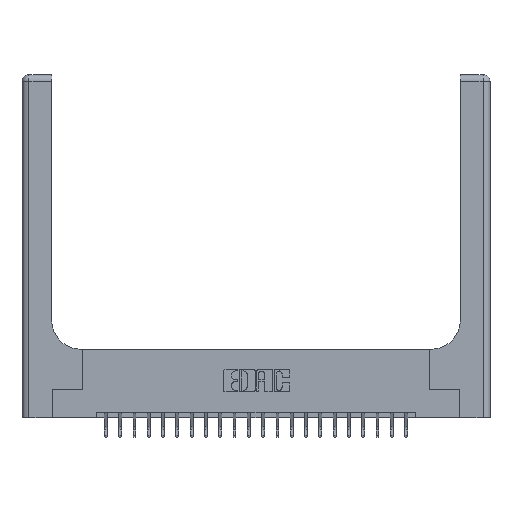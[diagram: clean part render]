
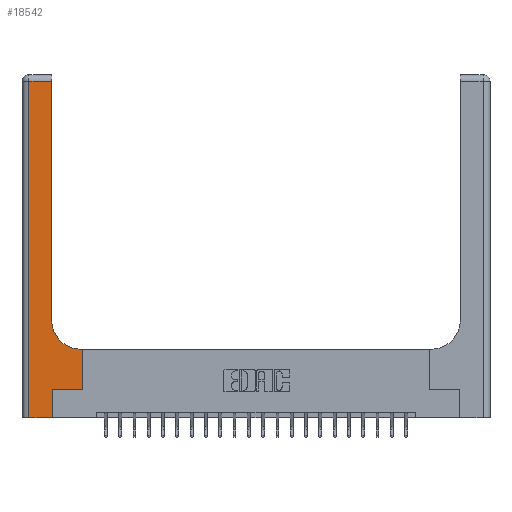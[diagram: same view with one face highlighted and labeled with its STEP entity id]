
A CAD part, top view. The second image highlights one B-rep face of the part: STEP entity #18542.
In plain terms, the highlighted planar face has unit normal (0, 0, 1).
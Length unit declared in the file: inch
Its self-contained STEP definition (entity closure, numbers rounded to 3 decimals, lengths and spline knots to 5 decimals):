
#567 = DIRECTION ( 'NONE',  ( -1., 0., 0. ) ) ;
#1198 = CARTESIAN_POINT ( 'NONE',  ( 0.528, 0.25, 0.37 ) ) ;
#1538 = EDGE_CURVE ( 'NONE', #21565, #9260, #12346, .T. ) ;
#1883 = FACE_OUTER_BOUND ( 'NONE', #14567, .T. ) ;
#2059 = EDGE_CURVE ( 'NONE', #5021, #21565, #5566, .T. ) ;
#2438 = ORIENTED_EDGE ( 'NONE', *, *, #4952, .T. ) ;
#3470 = CARTESIAN_POINT ( 'NONE',  ( 0.26, 3., 0.37 ) ) ;
#4332 = VERTEX_POINT ( 'NONE', #4841 ) ;
#4374 = LINE ( 'NONE', #22119, #8428 ) ;
#4595 = VERTEX_POINT ( 'NONE', #11902 ) ;
#4705 = DIRECTION ( 'NONE',  ( 0., -1., 0. ) ) ;
#4706 = VERTEX_POINT ( 'NONE', #13087 ) ;
#4841 = CARTESIAN_POINT ( 'NONE',  ( 0.06, 2.94, 0.37 ) ) ;
#4952 = EDGE_CURVE ( 'NONE', #4706, #21251, #4374, .T. ) ;
#5021 = VERTEX_POINT ( 'NONE', #15748 ) ;
#5566 = LINE ( 'NONE', #9264, #12848 ) ;
#5926 = ORIENTED_EDGE ( 'NONE', *, *, #2059, .T. ) ;
#6595 = PLANE ( 'NONE',  #22458 ) ;
#6806 = EDGE_CURVE ( 'NONE', #4332, #16799, #19696, .T. ) ;
#7234 = DIRECTION ( 'NONE',  ( 1., 0., 0. ) ) ;
#7977 = DIRECTION ( 'NONE',  ( 0., 1., 0. ) ) ;
#8107 = CARTESIAN_POINT ( 'NONE',  ( 0.06, 3., 0.37 ) ) ;
#8149 = VECTOR ( 'NONE', #17547, 39.37008 ) ;
#8370 = CARTESIAN_POINT ( 'NONE',  ( 0., 2.94, 0.37 ) ) ;
#8428 = VECTOR ( 'NONE', #13715, 39.37008 ) ;
#8444 = AXIS2_PLACEMENT_3D ( 'NONE', #10782, #17805, #7234 ) ;
#8693 = DIRECTION ( 'NONE',  ( 1., 0., 0. ) ) ;
#9260 = VERTEX_POINT ( 'NONE', #11089 ) ;
#9264 = CARTESIAN_POINT ( 'NONE',  ( 0.26, 0.6, 0.37 ) ) ;
#9341 = EDGE_CURVE ( 'NONE', #19269, #5021, #18955, .T. ) ;
#9403 = CARTESIAN_POINT ( 'NONE',  ( 0.51, 0.6, 0.37 ) ) ;
#9481 = EDGE_CURVE ( 'NONE', #16799, #4706, #19491, .T. ) ;
#10231 = EDGE_CURVE ( 'NONE', #9260, #4595, #22475, .T. ) ;
#10782 = CARTESIAN_POINT ( 'NONE',  ( 0.51, 0.85, 0.37 ) ) ;
#10850 = VECTOR ( 'NONE', #7977, 39.37008 ) ;
#10879 = ORIENTED_EDGE ( 'NONE', *, *, #20433, .T. ) ;
#11089 = CARTESIAN_POINT ( 'NONE',  ( 0.26, 0.85, 0.37 ) ) ;
#11902 = CARTESIAN_POINT ( 'NONE',  ( 0.26, 2.94, 0.37 ) ) ;
#12346 = CIRCLE ( 'NONE', #8444, 0.25 ) ;
#12388 = VECTOR ( 'NONE', #16835, 39.37008 ) ;
#12848 = VECTOR ( 'NONE', #567, 39.37008 ) ;
#13087 = CARTESIAN_POINT ( 'NONE',  ( 0.265, 0., 0.37 ) ) ;
#13192 = CARTESIAN_POINT ( 'NONE',  ( 0.06, 0., 0.37 ) ) ;
#13715 = DIRECTION ( 'NONE',  ( 0., 1., 0. ) ) ;
#13764 = DIRECTION ( 'NONE',  ( 0., 1., 0. ) ) ;
#14212 = EDGE_CURVE ( 'NONE', #21251, #19269, #14795, .T. ) ;
#14567 = EDGE_LOOP ( 'NONE', ( #18813, #10879, #17369, #20845, #2438, #21543, #15262, #5926, #15159 ) ) ;
#14571 = VECTOR ( 'NONE', #4705, 39.37008 ) ;
#14606 = VECTOR ( 'NONE', #13764, 39.37008 ) ;
#14795 = LINE ( 'NONE', #20562, #16419 ) ;
#15159 = ORIENTED_EDGE ( 'NONE', *, *, #1538, .T. ) ;
#15262 = ORIENTED_EDGE ( 'NONE', *, *, #9341, .T. ) ;
#15748 = CARTESIAN_POINT ( 'NONE',  ( 0.528, 0.6, 0.37 ) ) ;
#15886 = CARTESIAN_POINT ( 'NONE',  ( 0.265, 0.25, 0.37 ) ) ;
#16419 = VECTOR ( 'NONE', #8693, 39.37008 ) ;
#16799 = VERTEX_POINT ( 'NONE', #13192 ) ;
#16835 = DIRECTION ( 'NONE',  ( -1., 0., 0. ) ) ;
#17369 = ORIENTED_EDGE ( 'NONE', *, *, #6806, .T. ) ;
#17547 = DIRECTION ( 'NONE',  ( 1., 0., 0. ) ) ;
#17805 = DIRECTION ( 'NONE',  ( 0., 0., -1. ) ) ;
#18542 = ADVANCED_FACE ( 'NONE', ( #1883 ), #6595, .F. ) ;
#18679 = CARTESIAN_POINT ( 'NONE',  ( 0., 3., 0.37 ) ) ;
#18813 = ORIENTED_EDGE ( 'NONE', *, *, #10231, .T. ) ;
#18955 = LINE ( 'NONE', #1198, #10850 ) ;
#19269 = VERTEX_POINT ( 'NONE', #20668 ) ;
#19491 = LINE ( 'NONE', #20739, #8149 ) ;
#19696 = LINE ( 'NONE', #8107, #14571 ) ;
#19952 = LINE ( 'NONE', #8370, #12388 ) ;
#20274 = DIRECTION ( 'NONE',  ( -1., 0., 0. ) ) ;
#20423 = DIRECTION ( 'NONE',  ( 0., 0., -1. ) ) ;
#20433 = EDGE_CURVE ( 'NONE', #4595, #4332, #19952, .T. ) ;
#20562 = CARTESIAN_POINT ( 'NONE',  ( 0.265, 0.25, 0.37 ) ) ;
#20668 = CARTESIAN_POINT ( 'NONE',  ( 0.528, 0.25, 0.37 ) ) ;
#20739 = CARTESIAN_POINT ( 'NONE',  ( 0., 0., 0.37 ) ) ;
#20845 = ORIENTED_EDGE ( 'NONE', *, *, #9481, .T. ) ;
#21251 = VERTEX_POINT ( 'NONE', #15886 ) ;
#21543 = ORIENTED_EDGE ( 'NONE', *, *, #14212, .T. ) ;
#21565 = VERTEX_POINT ( 'NONE', #9403 ) ;
#22119 = CARTESIAN_POINT ( 'NONE',  ( 0.265, 0., 0.37 ) ) ;
#22458 = AXIS2_PLACEMENT_3D ( 'NONE', #18679, #20423, #20274 ) ;
#22475 = LINE ( 'NONE', #3470, #14606 ) ;
